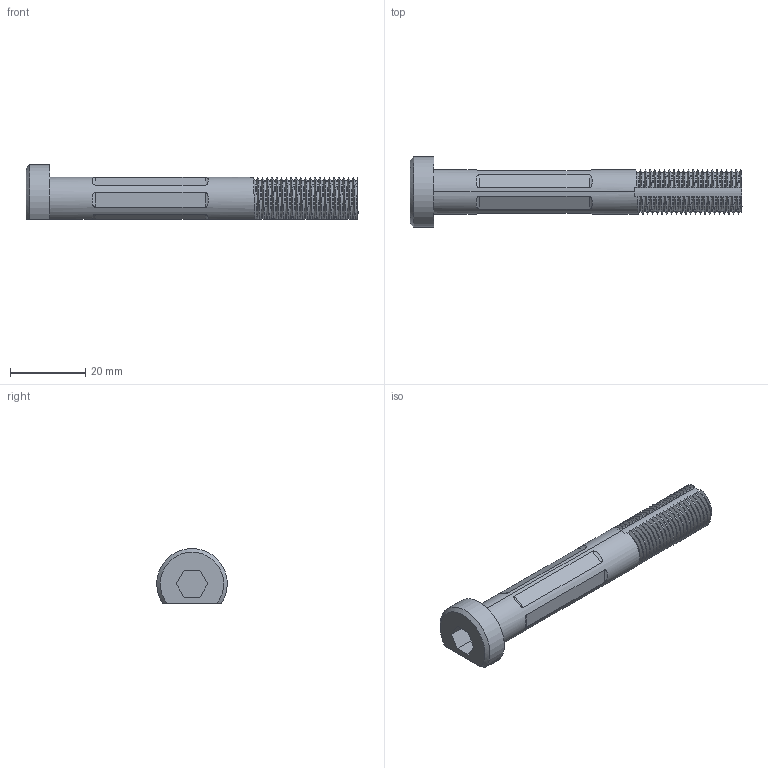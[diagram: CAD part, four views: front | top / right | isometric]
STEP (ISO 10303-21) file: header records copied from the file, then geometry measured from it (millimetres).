
FILE_DESCRIPTION (( 'STEP AP203' ), '1' );
FILE_NAME ('AF-HF-LR-PRT-007-STEP.STEP', '2020-10-04T16:14:20', ( '' ), ( '' ), 'SwSTEP 2.0', 'SolidWorks 2018', '' );
FILE_SCHEMA (( 'CONFIG_CONTROL_DESIGN' ));
Products named in the file (1): AF-HF-LR-PRT-007-STEP
Bounding box: 88.24 x 18.69 x 14.53 mm (x, y, z)
Volume: 9274.5 mm3; surface area: 4571.5 mm2
Topology: 1 solids, 1 shells, 238 faces, 679 edges, 448 vertices
Faces by surface type: bspline 134, cylinder 59, plane 44, cone 1
Entity records: 104770 total; most frequent: CARTESIAN_POINT 100306, ORIENTED_EDGE 1358, EDGE_CURVE 679, VERTEX_POINT 448, DIRECTION 431, EDGE_LOOP 243, FACE_OUTER_BOUND 238, ADVANCED_FACE 238
